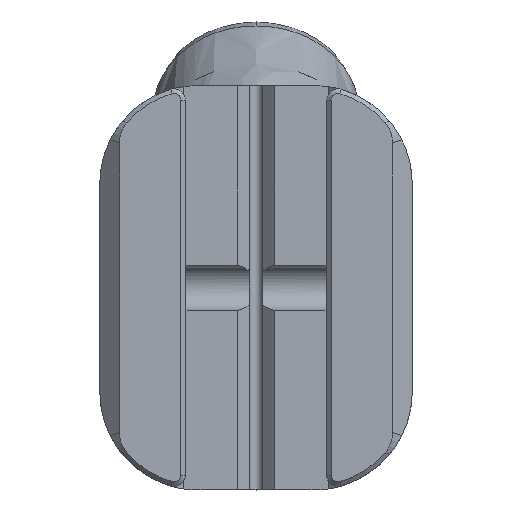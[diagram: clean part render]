
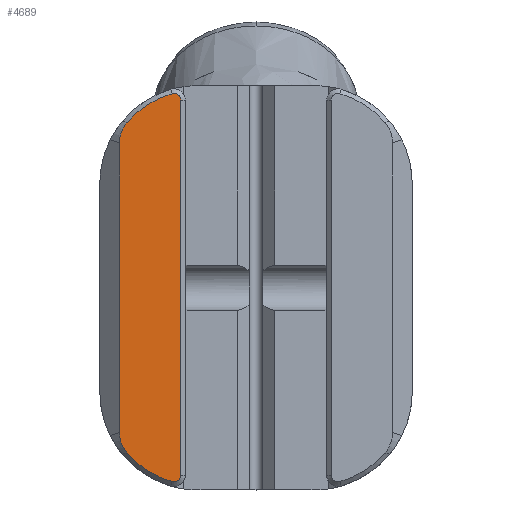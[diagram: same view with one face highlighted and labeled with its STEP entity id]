
A CAD part, top view. The second image highlights one B-rep face of the part: STEP entity #4689.
In plain terms, the highlighted planar face has unit normal (0, 0, 1).
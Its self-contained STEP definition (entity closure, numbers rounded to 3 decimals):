
#68=CIRCLE('',#5009,10.5);
#69=CIRCLE('',#5010,0.75);
#70=CIRCLE('',#5011,0.75);
#71=CIRCLE('',#5012,10.5);
#276=LINE('',#6111,#433);
#278=LINE('',#6128,#435);
#433=VECTOR('',#5306,10.);
#435=VECTOR('',#5318,10.);
#591=PLANE('',#5008);
#642=FACE_OUTER_BOUND('',#946,.T.);
#946=EDGE_LOOP('',(#2933,#2934,#2935,#2936,#2937,#2938,#2939,#2940));
#1253=B_SPLINE_CURVE_WITH_KNOTS('',3,(#6099,#6100,#6101,#6102,#6103,#6104),
 .UNSPECIFIED.,.F.,.F.,(4,2,4),(0.,0.128,0.255),
 .UNSPECIFIED.);
#1256=B_SPLINE_CURVE_WITH_KNOTS('',3,(#6133,#6134,#6135,#6136,#6137,#6138),
 .UNSPECIFIED.,.F.,.F.,(4,2,4),(0.,0.126,0.255),
 .UNSPECIFIED.);
#1668=VERTEX_POINT('',#6093);
#1669=VERTEX_POINT('',#6098);
#1670=VERTEX_POINT('',#6110);
#1674=VERTEX_POINT('',#6123);
#1675=VERTEX_POINT('',#6125);
#1676=VERTEX_POINT('',#6127);
#1677=VERTEX_POINT('',#6129);
#1678=VERTEX_POINT('',#6131);
#2145=EDGE_CURVE('',#1668,#1669,#1253,.T.);
#2147=EDGE_CURVE('',#1669,#1670,#276,.F.);
#2152=EDGE_CURVE('',#1674,#1668,#68,.T.);
#2153=EDGE_CURVE('',#1675,#1674,#69,.T.);
#2154=EDGE_CURVE('',#1676,#1675,#278,.T.);
#2155=EDGE_CURVE('',#1677,#1676,#70,.T.);
#2156=EDGE_CURVE('',#1678,#1677,#71,.T.);
#2157=EDGE_CURVE('',#1670,#1678,#1256,.T.);
#2933=ORIENTED_EDGE('',*,*,#2145,.F.);
#2934=ORIENTED_EDGE('',*,*,#2152,.F.);
#2935=ORIENTED_EDGE('',*,*,#2153,.F.);
#2936=ORIENTED_EDGE('',*,*,#2154,.F.);
#2937=ORIENTED_EDGE('',*,*,#2155,.F.);
#2938=ORIENTED_EDGE('',*,*,#2156,.F.);
#2939=ORIENTED_EDGE('',*,*,#2157,.F.);
#2940=ORIENTED_EDGE('',*,*,#2147,.F.);
#4689=ADVANCED_FACE('',(#642),#591,.F.);
#5008=AXIS2_PLACEMENT_3D('',#6122,#5312,#5313);
#5009=AXIS2_PLACEMENT_3D('',#6124,#5314,#5315);
#5010=AXIS2_PLACEMENT_3D('',#6126,#5316,#5317);
#5011=AXIS2_PLACEMENT_3D('',#6130,#5319,#5320);
#5012=AXIS2_PLACEMENT_3D('',#6132,#5321,#5322);
#5306=DIRECTION('',(0.,-1.,0.));
#5312=DIRECTION('center_axis',(0.,0.,
-1.));
#5313=DIRECTION('ref_axis',(1.,0.,0.));
#5314=DIRECTION('center_axis',(0.,0.,
-1.));
#5315=DIRECTION('ref_axis',(-0.707,-0.707,0.));
#5316=DIRECTION('center_axis',(0.,0.,
-1.));
#5317=DIRECTION('ref_axis',(0.602,-0.799,0.));
#5318=DIRECTION('',(0.,-1.,0.));
#5319=DIRECTION('center_axis',(0.,0.,
-1.));
#5320=DIRECTION('ref_axis',(0.602,0.799,0.));
#5321=DIRECTION('center_axis',(0.,0.,
-1.));
#5322=DIRECTION('ref_axis',(-0.707,0.707,0.));
#6093=CARTESIAN_POINT('',(-14.426,36.468,-6.092));
#6098=CARTESIAN_POINT('',(-15.293,38.787,-6.092));
#6099=CARTESIAN_POINT('Ctrl Pts',(-14.426,36.468,-6.092));
#6100=CARTESIAN_POINT('Ctrl Pts',(-14.707,36.791,-6.092));
#6101=CARTESIAN_POINT('Ctrl Pts',(-14.928,37.156,-6.092));
#6102=CARTESIAN_POINT('Ctrl Pts',(-15.223,37.952,-6.092));
#6103=CARTESIAN_POINT('Ctrl Pts',(-15.293,38.366,-6.092));
#6104=CARTESIAN_POINT('Ctrl Pts',(-15.293,38.787,-6.092));
#6110=CARTESIAN_POINT('',(-15.293,71.221,-6.092));
#6111=CARTESIAN_POINT('',(-15.293,69.903,-6.092));
#6122=CARTESIAN_POINT('Origin',(-20.269,69.903,-6.092));
#6123=CARTESIAN_POINT('',(-9.393,33.261,-6.092));
#6124=CARTESIAN_POINT('Origin',(-6.5,43.355,-6.092));
#6125=CARTESIAN_POINT('',(-8.436,33.982,-6.092));
#6126=CARTESIAN_POINT('Origin',(-9.186,33.982,-6.092));
#6127=CARTESIAN_POINT('',(-8.436,76.026,-6.092));
#6128=CARTESIAN_POINT('',(-8.436,42.504,-6.092));
#6129=CARTESIAN_POINT('',(-9.393,76.747,-6.092));
#6130=CARTESIAN_POINT('Origin',(-9.186,76.026,-6.092));
#6131=CARTESIAN_POINT('',(-14.426,73.539,-6.092));
#6132=CARTESIAN_POINT('Origin',(-6.5,66.653,-6.092));
#6133=CARTESIAN_POINT('Ctrl Pts',(-15.293,71.221,-6.092));
#6134=CARTESIAN_POINT('Ctrl Pts',(-15.293,71.642,-6.092));
#6135=CARTESIAN_POINT('Ctrl Pts',(-15.223,72.055,-6.092));
#6136=CARTESIAN_POINT('Ctrl Pts',(-14.928,72.851,-6.092));
#6137=CARTESIAN_POINT('Ctrl Pts',(-14.707,73.216,-6.092));
#6138=CARTESIAN_POINT('Ctrl Pts',(-14.426,73.539,-6.092));
